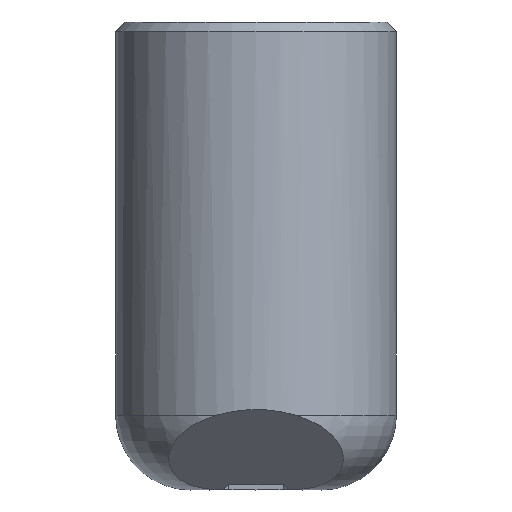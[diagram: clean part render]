
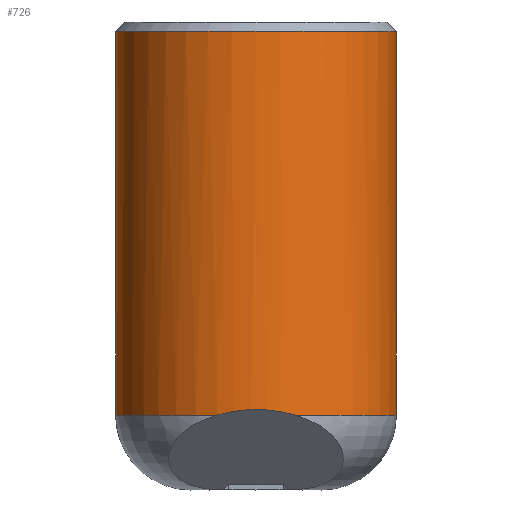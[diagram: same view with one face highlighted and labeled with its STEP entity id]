
A CAD part, front view. The second image highlights one B-rep face of the part: STEP entity #726.
In plain terms, the highlighted cylindrical face has radius 7.5 mm (diameter 15 mm), a partial arc.
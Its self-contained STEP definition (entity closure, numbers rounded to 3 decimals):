
#17 = AXIS2_PLACEMENT_3D ( 'NONE', #546, #735, #419 ) ;
#25 = CARTESIAN_POINT ( 'NONE',  ( -7.5, 0., 25. ) ) ;
#34 = EDGE_CURVE ( 'NONE', #825, #129, #74, .T. ) ;
#39 = VERTEX_POINT ( 'NONE', #475 ) ;
#40 = VECTOR ( 'NONE', #761, 1000. ) ;
#49 = EDGE_CURVE ( 'NONE', #39, #825, #274, .T. ) ;
#68 = DIRECTION ( 'NONE',  ( 0., 0., -1. ) ) ;
#71 = DIRECTION ( 'NONE',  ( 0., 0., 1. ) ) ;
#74 = CIRCLE ( 'NONE', #660, 7.5 ) ;
#93 = FACE_OUTER_BOUND ( 'NONE', #663, .T. ) ;
#110 = DIRECTION ( 'NONE',  ( 0., 0., -1. ) ) ;
#129 = VERTEX_POINT ( 'NONE', #594 ) ;
#134 = CARTESIAN_POINT ( 'NONE',  ( 0., 0., 4. ) ) ;
#166 = CARTESIAN_POINT ( 'NONE',  ( 0., 0., 25. ) ) ;
#190 = VECTOR ( 'NONE', #68, 1000. ) ;
#202 = ORIENTED_EDGE ( 'NONE', *, *, #505, .F. ) ;
#216 = CARTESIAN_POINT ( 'NONE',  ( 2.096, -7.201, 4. ) ) ;
#225 = CARTESIAN_POINT ( 'NONE',  ( 7.5, 0., 25. ) ) ;
#234 = CARTESIAN_POINT ( 'NONE',  ( -2.096, -7.201, 4. ) ) ;
#265 = VERTEX_POINT ( 'NONE', #216 ) ;
#274 = LINE ( 'NONE', #25, #190 ) ;
#298 = EDGE_CURVE ( 'NONE', #373, #39, #506, .T. ) ;
#307 = CARTESIAN_POINT ( 'NONE',  ( 0., 0., 24.5 ) ) ;
#347 = AXIS2_PLACEMENT_3D ( 'NONE', #166, #110, #692 ) ;
#349 = CYLINDRICAL_SURFACE ( 'NONE', #347, 7.5 ) ;
#373 = VERTEX_POINT ( 'NONE', #643 ) ;
#384 = CARTESIAN_POINT ( 'NONE',  ( -7.5, 0., 4. ) ) ;
#390 = ORIENTED_EDGE ( 'NONE', *, *, #49, .T. ) ;
#392 =( BOUNDED_CURVE ( )  B_SPLINE_CURVE ( 3, ( #234, #706, #496, #753 ),
 .UNSPECIFIED., .F., .F. ) 
 B_SPLINE_CURVE_WITH_KNOTS ( ( 4, 4 ),
 ( 2.858, 3.425 ),
 .UNSPECIFIED. ) 
 CURVE ( )  GEOMETRIC_REPRESENTATION_ITEM ( )  RATIONAL_B_SPLINE_CURVE ( ( 1., 0.973, 0.973, 1. ) ) 
 REPRESENTATION_ITEM ( '' )  );
#399 = DIRECTION ( 'NONE',  ( 1., 0., 0. ) ) ;
#419 = DIRECTION ( 'NONE',  ( 1., 0., 0. ) ) ;
#440 = DIRECTION ( 'NONE',  ( 0., 0., -1. ) ) ;
#475 = CARTESIAN_POINT ( 'NONE',  ( -7.5, 0., 24.5 ) ) ;
#484 = EDGE_CURVE ( 'NONE', #265, #739, #627, .T. ) ;
#496 = CARTESIAN_POINT ( 'NONE',  ( 0.718, -7.602, 4.403 ) ) ;
#498 = EDGE_CURVE ( 'NONE', #129, #265, #392, .T. ) ;
#499 = DIRECTION ( 'NONE',  ( 1., 0., 0. ) ) ;
#505 = EDGE_CURVE ( 'NONE', #373, #739, #550, .T. ) ;
#506 = CIRCLE ( 'NONE', #705, 7.5 ) ;
#527 = ORIENTED_EDGE ( 'NONE', *, *, #298, .T. ) ;
#546 = CARTESIAN_POINT ( 'NONE',  ( 0., 0., 4. ) ) ;
#550 = LINE ( 'NONE', #225, #40 ) ;
#594 = CARTESIAN_POINT ( 'NONE',  ( -2.096, -7.201, 4. ) ) ;
#617 = CARTESIAN_POINT ( 'NONE',  ( 7.5, 0., 4. ) ) ;
#627 = CIRCLE ( 'NONE', #17, 7.5 ) ;
#643 = CARTESIAN_POINT ( 'NONE',  ( 7.5, 0., 24.5 ) ) ;
#660 = AXIS2_PLACEMENT_3D ( 'NONE', #134, #71, #399 ) ;
#663 = EDGE_LOOP ( 'NONE', ( #202, #527, #390, #796, #788, #733 ) ) ;
#692 = DIRECTION ( 'NONE',  ( -1., 0., 0. ) ) ;
#705 = AXIS2_PLACEMENT_3D ( 'NONE', #307, #440, #499 ) ;
#706 = CARTESIAN_POINT ( 'NONE',  ( -0.718, -7.602, 4.403 ) ) ;
#726 = ADVANCED_FACE ( 'NONE', ( #93 ), #349, .T. ) ;
#733 = ORIENTED_EDGE ( 'NONE', *, *, #484, .T. ) ;
#735 = DIRECTION ( 'NONE',  ( 0., 0., 1. ) ) ;
#739 = VERTEX_POINT ( 'NONE', #617 ) ;
#753 = CARTESIAN_POINT ( 'NONE',  ( 2.096, -7.201, 4. ) ) ;
#761 = DIRECTION ( 'NONE',  ( 0., 0., -1. ) ) ;
#788 = ORIENTED_EDGE ( 'NONE', *, *, #498, .T. ) ;
#796 = ORIENTED_EDGE ( 'NONE', *, *, #34, .T. ) ;
#825 = VERTEX_POINT ( 'NONE', #384 ) ;
